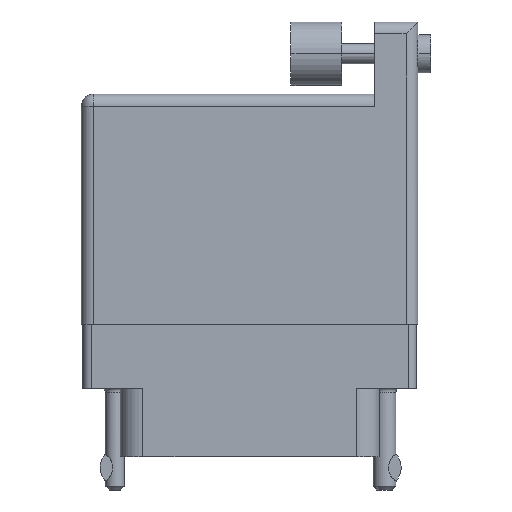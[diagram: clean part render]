
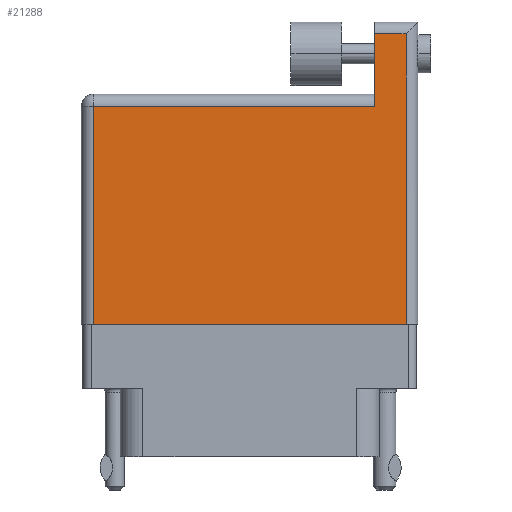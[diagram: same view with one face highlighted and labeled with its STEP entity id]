
A CAD part, front view. The second image highlights one B-rep face of the part: STEP entity #21288.
In plain terms, the highlighted face is planar.
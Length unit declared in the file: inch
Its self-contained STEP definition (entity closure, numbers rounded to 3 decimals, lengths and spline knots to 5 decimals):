
#495 = EDGE_CURVE ( 'NONE', #35026, #27616, #929, .T. ) ;
#902 = CARTESIAN_POINT ( 'NONE',  ( 1.278, 1.19, 0. ) ) ;
#929 = LINE ( 'NONE', #1107, #24499 ) ;
#1107 = CARTESIAN_POINT ( 'NONE',  ( 1.155, 1.19, 0. ) ) ;
#1572 = ORIENTED_EDGE ( 'NONE', *, *, #495, .T. ) ;
#2238 = CARTESIAN_POINT ( 'NONE',  ( 1.278, 1.143, 0. ) ) ;
#2244 = CARTESIAN_POINT ( 'NONE',  ( 1.278, 0., 0. ) ) ;
#2414 = DIRECTION ( 'NONE',  ( -1., 0., 0. ) ) ;
#3801 = EDGE_LOOP ( 'NONE', ( #9099, #17963, #17462, #1572, #35008, #9241 ) ) ;
#4303 = DIRECTION ( 'NONE',  ( -1., 0., 0. ) ) ;
#4942 = CARTESIAN_POINT ( 'NONE',  ( 0.047, 0.859, 0. ) ) ;
#5152 = VERTEX_POINT ( 'NONE', #2238 ) ;
#6093 = EDGE_CURVE ( 'NONE', #20474, #5152, #6655, .T. ) ;
#6655 = LINE ( 'NONE', #902, #15062 ) ;
#7458 = DIRECTION ( 'NONE',  ( -1., 0., 0. ) ) ;
#7656 = LINE ( 'NONE', #18669, #10504 ) ;
#8028 = VERTEX_POINT ( 'NONE', #4942 ) ;
#8961 = CARTESIAN_POINT ( 'NONE',  ( 1.155, 1.143, 0. ) ) ;
#9099 = ORIENTED_EDGE ( 'NONE', *, *, #23293, .T. ) ;
#9241 = ORIENTED_EDGE ( 'NONE', *, *, #24413, .T. ) ;
#10219 = DIRECTION ( 'NONE',  ( 0., -1., 0. ) ) ;
#10504 = VECTOR ( 'NONE', #13444, 39.37008 ) ;
#11769 = DIRECTION ( 'NONE',  ( 0., -1., 0. ) ) ;
#12374 = CARTESIAN_POINT ( 'NONE',  ( 1.155, 0.859, 0. ) ) ;
#13444 = DIRECTION ( 'NONE',  ( 1., 0., 0. ) ) ;
#13603 = LINE ( 'NONE', #24617, #31486 ) ;
#13708 = AXIS2_PLACEMENT_3D ( 'NONE', #31791, #29237, #4303 ) ;
#15062 = VECTOR ( 'NONE', #28700, 39.37008 ) ;
#15527 = PLANE ( 'NONE',  #13708 ) ;
#15639 = LINE ( 'NONE', #17968, #26704 ) ;
#15713 = CARTESIAN_POINT ( 'NONE',  ( 0.047, 0., 0. ) ) ;
#16140 = LINE ( 'NONE', #27153, #31002 ) ;
#17462 = ORIENTED_EDGE ( 'NONE', *, *, #31863, .T. ) ;
#17963 = ORIENTED_EDGE ( 'NONE', *, *, #6093, .T. ) ;
#17968 = CARTESIAN_POINT ( 'NONE',  ( 0.047, 0., 0. ) ) ;
#18669 = CARTESIAN_POINT ( 'NONE',  ( 0., 0., 0. ) ) ;
#20474 = VERTEX_POINT ( 'NONE', #2244 ) ;
#20548 = EDGE_CURVE ( 'NONE', #27616, #8028, #16140, .T. ) ;
#21288 = ADVANCED_FACE ( 'NONE', ( #31617 ), #15527, .F. ) ;
#23293 = EDGE_CURVE ( 'NONE', #28715, #20474, #7656, .T. ) ;
#24413 = EDGE_CURVE ( 'NONE', #8028, #28715, #15639, .T. ) ;
#24499 = VECTOR ( 'NONE', #11769, 39.37008 ) ;
#24617 = CARTESIAN_POINT ( 'NONE',  ( 1.155, 1.143, 0. ) ) ;
#26704 = VECTOR ( 'NONE', #10219, 39.37008 ) ;
#27153 = CARTESIAN_POINT ( 'NONE',  ( 0., 0.859, 0. ) ) ;
#27616 = VERTEX_POINT ( 'NONE', #12374 ) ;
#28700 = DIRECTION ( 'NONE',  ( 0., 1., 0. ) ) ;
#28715 = VERTEX_POINT ( 'NONE', #15713 ) ;
#29237 = DIRECTION ( 'NONE',  ( 0., 0., -1. ) ) ;
#31002 = VECTOR ( 'NONE', #2414, 39.37008 ) ;
#31486 = VECTOR ( 'NONE', #7458, 39.37008 ) ;
#31617 = FACE_OUTER_BOUND ( 'NONE', #3801, .T. ) ;
#31791 = CARTESIAN_POINT ( 'NONE',  ( 0., 0.906, 0. ) ) ;
#31863 = EDGE_CURVE ( 'NONE', #5152, #35026, #13603, .T. ) ;
#35008 = ORIENTED_EDGE ( 'NONE', *, *, #20548, .T. ) ;
#35026 = VERTEX_POINT ( 'NONE', #8961 ) ;
